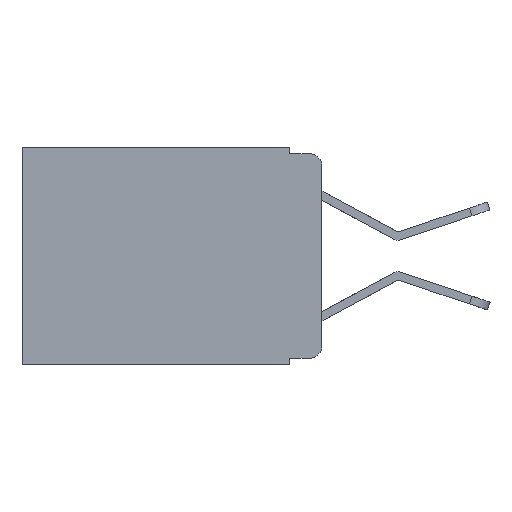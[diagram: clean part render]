
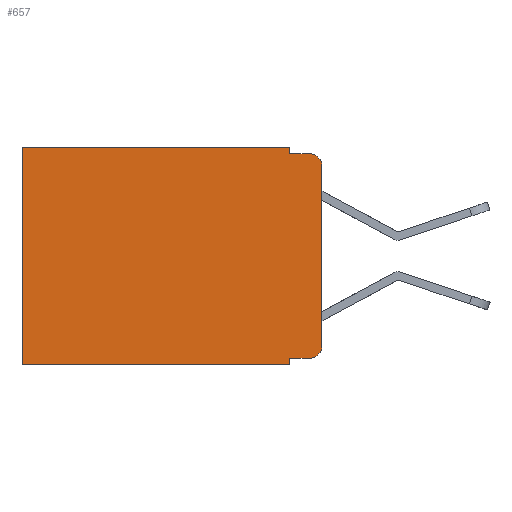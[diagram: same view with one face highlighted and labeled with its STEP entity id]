
A CAD part, left-side view. The second image highlights one B-rep face of the part: STEP entity #657.
In plain terms, the highlighted planar face has unit normal (-1, 0, 0).
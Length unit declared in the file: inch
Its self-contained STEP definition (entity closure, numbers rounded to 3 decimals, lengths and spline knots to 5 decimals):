
#10 = ORIENTED_EDGE ( 'NONE', *, *, #12838, .T. ) ;
#18 = CARTESIAN_POINT ( 'NONE',  ( 0.298, 0.02, -0.01 ) ) ;
#359 = LINE ( 'NONE', #3549, #11771 ) ;
#444 = VECTOR ( 'NONE', #6785, 39.37008 ) ;
#611 = DIRECTION ( 'NONE',  ( 1., 0., 0. ) ) ;
#630 = VERTEX_POINT ( 'NONE', #9668 ) ;
#637 = CARTESIAN_POINT ( 'NONE',  ( 0.298, 0.051, -0.333 ) ) ;
#657 = ADVANCED_FACE ( 'NONE', ( #5671 ), #3653, .F. ) ;
#918 = DIRECTION ( 'NONE',  ( 0., 0., -1. ) ) ;
#939 = VECTOR ( 'NONE', #3962, 39.37008 ) ;
#965 = LINE ( 'NONE', #5016, #9519 ) ;
#993 = ORIENTED_EDGE ( 'NONE', *, *, #10595, .T. ) ;
#1175 = ORIENTED_EDGE ( 'NONE', *, *, #8537, .T. ) ;
#1660 = CARTESIAN_POINT ( 'NONE',  ( 0.298, 0., 0. ) ) ;
#1867 = CARTESIAN_POINT ( 'NONE',  ( 0.298, 0.02, -0.313 ) ) ;
#2285 = EDGE_CURVE ( 'NONE', #9331, #11290, #7977, .T. ) ;
#2416 = AXIS2_PLACEMENT_3D ( 'NONE', #4528, #611, #9609 ) ;
#2607 = LINE ( 'NONE', #12493, #11311 ) ;
#2822 = VERTEX_POINT ( 'NONE', #12839 ) ;
#2985 = CARTESIAN_POINT ( 'NONE',  ( 0.298, 0.02, -0.03 ) ) ;
#2997 = CARTESIAN_POINT ( 'NONE',  ( 0.298, 0.051, -0.01 ) ) ;
#3398 = VECTOR ( 'NONE', #5625, 39.37008 ) ;
#3418 = DIRECTION ( 'NONE',  ( 0., 1., 0. ) ) ;
#3536 = ORIENTED_EDGE ( 'NONE', *, *, #13095, .F. ) ;
#3549 = CARTESIAN_POINT ( 'NONE',  ( 0.298, 0., -0.343 ) ) ;
#3653 = PLANE ( 'NONE',  #2416 ) ;
#3895 = CARTESIAN_POINT ( 'NONE',  ( 0.298, 0., 0. ) ) ;
#3962 = DIRECTION ( 'NONE',  ( 0., 1., 0. ) ) ;
#3989 = CARTESIAN_POINT ( 'NONE',  ( 0.298, 0.051, -0.01 ) ) ;
#4177 = VERTEX_POINT ( 'NONE', #12843 ) ;
#4511 = VECTOR ( 'NONE', #11582, 39.37008 ) ;
#4528 = CARTESIAN_POINT ( 'NONE',  ( 0.298, 0., 0. ) ) ;
#4617 = EDGE_CURVE ( 'NONE', #10686, #4825, #965, .T. ) ;
#4729 = AXIS2_PLACEMENT_3D ( 'NONE', #2985, #10038, #918 ) ;
#4825 = VERTEX_POINT ( 'NONE', #9558 ) ;
#4950 = EDGE_LOOP ( 'NONE', ( #12263, #993, #11938, #8941, #8242, #1175, #3536, #8139, #10, #5906 ) ) ;
#5016 = CARTESIAN_POINT ( 'NONE',  ( 0.298, 0.051, 0. ) ) ;
#5625 = DIRECTION ( 'NONE',  ( 0., 0., -1. ) ) ;
#5671 = FACE_OUTER_BOUND ( 'NONE', #4950, .T. ) ;
#5892 = CARTESIAN_POINT ( 'NONE',  ( 0.298, 0.051, 0. ) ) ;
#5906 = ORIENTED_EDGE ( 'NONE', *, *, #7419, .T. ) ;
#6127 = CARTESIAN_POINT ( 'NONE',  ( 0.298, 0.051, 0. ) ) ;
#6247 = EDGE_CURVE ( 'NONE', #9331, #6549, #8745, .T. ) ;
#6319 = CARTESIAN_POINT ( 'NONE',  ( 0.298, 0.473, 0. ) ) ;
#6487 = DIRECTION ( 'NONE',  ( 0., 0., -1. ) ) ;
#6549 = VERTEX_POINT ( 'NONE', #2997 ) ;
#6620 = AXIS2_PLACEMENT_3D ( 'NONE', #1867, #12012, #8784 ) ;
#6785 = DIRECTION ( 'NONE',  ( 0., -1., 0. ) ) ;
#7131 = CARTESIAN_POINT ( 'NONE',  ( 0.298, 0.051, -0.333 ) ) ;
#7221 = CARTESIAN_POINT ( 'NONE',  ( 0.298, 0., -0.313 ) ) ;
#7249 = DIRECTION ( 'NONE',  ( 0., 0., -1. ) ) ;
#7419 = EDGE_CURVE ( 'NONE', #2822, #10271, #12314, .T. ) ;
#7451 = EDGE_CURVE ( 'NONE', #6549, #7900, #9919, .T. ) ;
#7779 = DIRECTION ( 'NONE',  ( 0., -1., 0. ) ) ;
#7900 = VERTEX_POINT ( 'NONE', #18 ) ;
#7977 = LINE ( 'NONE', #3895, #939 ) ;
#8139 = ORIENTED_EDGE ( 'NONE', *, *, #4617, .F. ) ;
#8242 = ORIENTED_EDGE ( 'NONE', *, *, #2285, .T. ) ;
#8537 = EDGE_CURVE ( 'NONE', #11290, #4177, #2607, .T. ) ;
#8545 = EDGE_CURVE ( 'NONE', #630, #10271, #11510, .T. ) ;
#8745 = LINE ( 'NONE', #5892, #3398 ) ;
#8784 = DIRECTION ( 'NONE',  ( 0., 0., -1. ) ) ;
#8941 = ORIENTED_EDGE ( 'NONE', *, *, #6247, .F. ) ;
#8997 = CIRCLE ( 'NONE', #4729, 0.02 ) ;
#9331 = VERTEX_POINT ( 'NONE', #6127 ) ;
#9519 = VECTOR ( 'NONE', #7249, 39.37008 ) ;
#9558 = CARTESIAN_POINT ( 'NONE',  ( 0.298, 0.051, -0.343 ) ) ;
#9609 = DIRECTION ( 'NONE',  ( 0., 0., -1. ) ) ;
#9668 = CARTESIAN_POINT ( 'NONE',  ( 0.298, 0., -0.03 ) ) ;
#9919 = LINE ( 'NONE', #3989, #444 ) ;
#10038 = DIRECTION ( 'NONE',  ( -1., 0., 0. ) ) ;
#10271 = VERTEX_POINT ( 'NONE', #7221 ) ;
#10595 = EDGE_CURVE ( 'NONE', #630, #7900, #8997, .T. ) ;
#10686 = VERTEX_POINT ( 'NONE', #7131 ) ;
#11290 = VERTEX_POINT ( 'NONE', #6319 ) ;
#11311 = VECTOR ( 'NONE', #6487, 39.37008 ) ;
#11510 = LINE ( 'NONE', #1660, #4511 ) ;
#11582 = DIRECTION ( 'NONE',  ( 0., 0., -1. ) ) ;
#11624 = VECTOR ( 'NONE', #7779, 39.37008 ) ;
#11771 = VECTOR ( 'NONE', #3418, 39.37008 ) ;
#11938 = ORIENTED_EDGE ( 'NONE', *, *, #7451, .F. ) ;
#12012 = DIRECTION ( 'NONE',  ( -1., 0., 0. ) ) ;
#12049 = LINE ( 'NONE', #637, #11624 ) ;
#12263 = ORIENTED_EDGE ( 'NONE', *, *, #8545, .F. ) ;
#12314 = CIRCLE ( 'NONE', #6620, 0.02 ) ;
#12493 = CARTESIAN_POINT ( 'NONE',  ( 0.298, 0.473, 0. ) ) ;
#12838 = EDGE_CURVE ( 'NONE', #10686, #2822, #12049, .T. ) ;
#12839 = CARTESIAN_POINT ( 'NONE',  ( 0.298, 0.02, -0.333 ) ) ;
#12843 = CARTESIAN_POINT ( 'NONE',  ( 0.298, 0.473, -0.343 ) ) ;
#13095 = EDGE_CURVE ( 'NONE', #4825, #4177, #359, .T. ) ;
